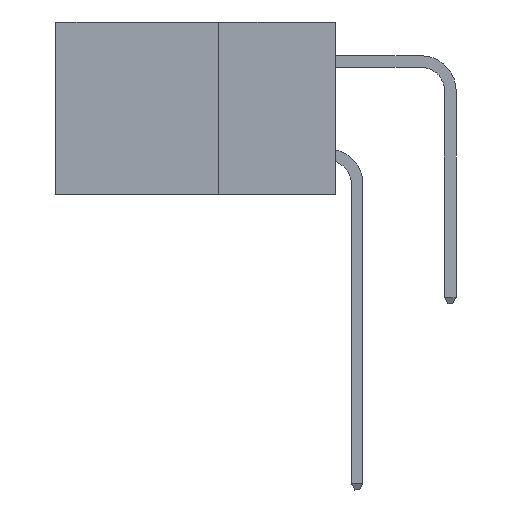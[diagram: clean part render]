
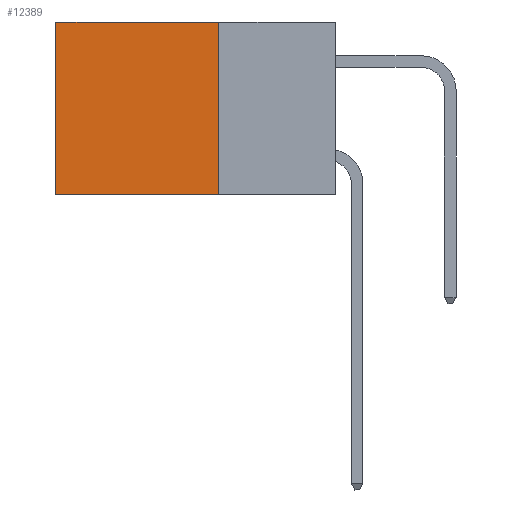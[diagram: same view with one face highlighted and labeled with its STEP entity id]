
A CAD part, left-side view. The second image highlights one B-rep face of the part: STEP entity #12389.
In plain terms, the highlighted planar face has unit normal (-1, 0, 0).
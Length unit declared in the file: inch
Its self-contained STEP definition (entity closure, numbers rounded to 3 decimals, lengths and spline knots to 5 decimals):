
#803 = CARTESIAN_POINT ( 'NONE',  ( 0.2875, 0.25, 0. ) ) ;
#898 = DIRECTION ( 'NONE',  ( 0., 1., 0. ) ) ;
#1889 = VECTOR ( 'NONE', #13875, 39.37008 ) ;
#1923 = CARTESIAN_POINT ( 'NONE',  ( 0.2875, 0.6, 0. ) ) ;
#2121 = CARTESIAN_POINT ( 'NONE',  ( 0.2875, 0.25, -0.37 ) ) ;
#2663 = LINE ( 'NONE', #2121, #11356 ) ;
#3140 = DIRECTION ( 'NONE',  ( 0., 0., -1. ) ) ;
#3279 = DIRECTION ( 'NONE',  ( 0., 0., -1. ) ) ;
#3338 = ORIENTED_EDGE ( 'NONE', *, *, #3736, .T. ) ;
#3736 = EDGE_CURVE ( 'NONE', #10071, #11960, #8082, .T. ) ;
#4038 = FACE_OUTER_BOUND ( 'NONE', #13729, .T. ) ;
#4160 = EDGE_CURVE ( 'NONE', #6607, #9847, #2663, .T. ) ;
#4436 = PLANE ( 'NONE',  #7987 ) ;
#5566 = EDGE_CURVE ( 'NONE', #11960, #9847, #10615, .T. ) ;
#6019 = CARTESIAN_POINT ( 'NONE',  ( 0.2875, 0.6, 0. ) ) ;
#6607 = VERTEX_POINT ( 'NONE', #14199 ) ;
#7190 = CARTESIAN_POINT ( 'NONE',  ( 0.2875, 0.25, 0. ) ) ;
#7542 = CARTESIAN_POINT ( 'NONE',  ( 0.2875, 0.25, 0. ) ) ;
#7682 = VECTOR ( 'NONE', #3140, 39.37008 ) ;
#7958 = DIRECTION ( 'NONE',  ( 0., 0., -1. ) ) ;
#7987 = AXIS2_PLACEMENT_3D ( 'NONE', #803, #10088, #3279 ) ;
#8082 = LINE ( 'NONE', #7190, #1889 ) ;
#8281 = VECTOR ( 'NONE', #7958, 39.37008 ) ;
#8519 = ORIENTED_EDGE ( 'NONE', *, *, #5566, .T. ) ;
#8610 = LINE ( 'NONE', #13523, #8281 ) ;
#9406 = CARTESIAN_POINT ( 'NONE',  ( 0.2875, 0.6, -0.37 ) ) ;
#9847 = VERTEX_POINT ( 'NONE', #9406 ) ;
#10071 = VERTEX_POINT ( 'NONE', #7542 ) ;
#10088 = DIRECTION ( 'NONE',  ( 1., 0., 0. ) ) ;
#10615 = LINE ( 'NONE', #1923, #7682 ) ;
#11356 = VECTOR ( 'NONE', #898, 39.37008 ) ;
#11960 = VERTEX_POINT ( 'NONE', #6019 ) ;
#12389 = ADVANCED_FACE ( 'NONE', ( #4038 ), #4436, .F. ) ;
#12672 = ORIENTED_EDGE ( 'NONE', *, *, #4160, .F. ) ;
#13361 = ORIENTED_EDGE ( 'NONE', *, *, #14242, .F. ) ;
#13523 = CARTESIAN_POINT ( 'NONE',  ( 0.2875, 0.25, 0. ) ) ;
#13729 = EDGE_LOOP ( 'NONE', ( #8519, #12672, #13361, #3338 ) ) ;
#13875 = DIRECTION ( 'NONE',  ( 0., 1., 0. ) ) ;
#14199 = CARTESIAN_POINT ( 'NONE',  ( 0.2875, 0.25, -0.37 ) ) ;
#14242 = EDGE_CURVE ( 'NONE', #10071, #6607, #8610, .T. ) ;
